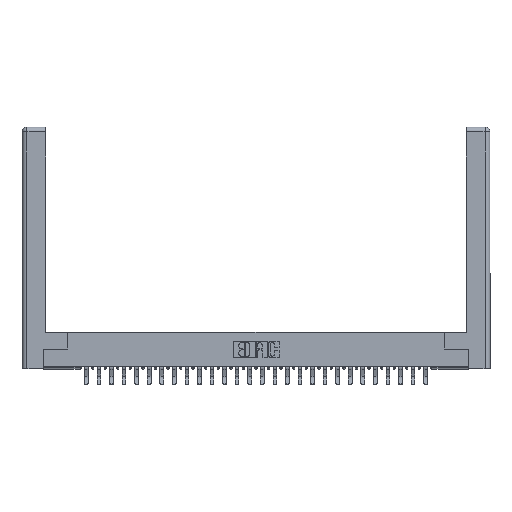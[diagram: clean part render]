
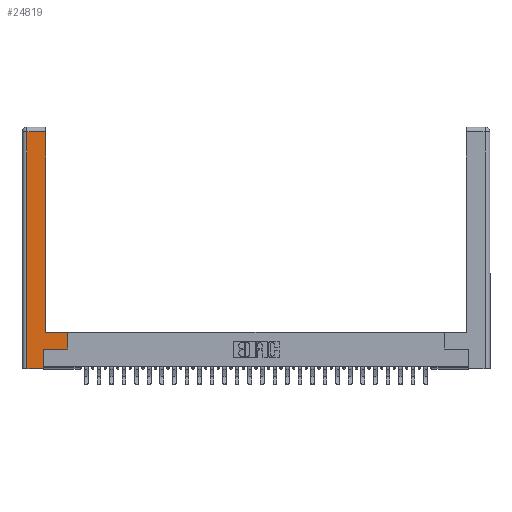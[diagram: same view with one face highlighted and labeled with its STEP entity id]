
A CAD part, top view. The second image highlights one B-rep face of the part: STEP entity #24819.
In plain terms, the highlighted planar face has unit normal (0, 0, 1).
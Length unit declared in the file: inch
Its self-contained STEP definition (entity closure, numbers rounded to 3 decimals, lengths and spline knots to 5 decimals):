
#255 = FACE_OUTER_BOUND ( 'NONE', #34238, .T. ) ;
#526 = DIRECTION ( 'NONE',  ( 0., 0., -1. ) ) ;
#2604 = CARTESIAN_POINT ( 'NONE',  ( 0., 0., 0. ) ) ;
#2842 = VECTOR ( 'NONE', #16489, 39.37008 ) ;
#3106 = ORIENTED_EDGE ( 'NONE', *, *, #4891, .T. ) ;
#4141 = CARTESIAN_POINT ( 'NONE',  ( 0.565, 0.45, 0. ) ) ;
#4891 = EDGE_CURVE ( 'NONE', #26411, #34265, #20602, .T. ) ;
#5141 = DIRECTION ( 'NONE',  ( -1., 0., 0. ) ) ;
#5194 = VERTEX_POINT ( 'NONE', #5573 ) ;
#5537 = PLANE ( 'NONE',  #10053 ) ;
#5573 = CARTESIAN_POINT ( 'NONE',  ( 0.565, 0.245, 0. ) ) ;
#6093 = VECTOR ( 'NONE', #22585, 39.37008 ) ;
#6288 = CARTESIAN_POINT ( 'NONE',  ( 0.295, 0.45, 0. ) ) ;
#7735 = CARTESIAN_POINT ( 'NONE',  ( 0.295, 0.45, 0. ) ) ;
#8131 = CARTESIAN_POINT ( 'NONE',  ( 0.0615, 0., 0. ) ) ;
#9075 = ORIENTED_EDGE ( 'NONE', *, *, #29049, .T. ) ;
#9185 = VECTOR ( 'NONE', #31605, 39.37008 ) ;
#9565 = CARTESIAN_POINT ( 'NONE',  ( 0.0615, 2.94, 0. ) ) ;
#10053 = AXIS2_PLACEMENT_3D ( 'NONE', #2604, #526, #26789 ) ;
#10129 = VERTEX_POINT ( 'NONE', #15245 ) ;
#10498 = LINE ( 'NONE', #4141, #15585 ) ;
#11147 = ORIENTED_EDGE ( 'NONE', *, *, #16006, .T. ) ;
#11263 = CARTESIAN_POINT ( 'NONE',  ( 0.295, 2.94, 0. ) ) ;
#12199 = ORIENTED_EDGE ( 'NONE', *, *, #34478, .T. ) ;
#12712 = CARTESIAN_POINT ( 'NONE',  ( 0.565, 0.245, 0. ) ) ;
#14322 = CARTESIAN_POINT ( 'NONE',  ( 0.0615, 0., 0. ) ) ;
#14647 = LINE ( 'NONE', #8131, #2842 ) ;
#14745 = CARTESIAN_POINT ( 'NONE',  ( 0.265, 0.245, 0. ) ) ;
#15245 = CARTESIAN_POINT ( 'NONE',  ( 0.565, 0.45, 0. ) ) ;
#15457 = EDGE_CURVE ( 'NONE', #34265, #28765, #17475, .T. ) ;
#15585 = VECTOR ( 'NONE', #33820, 39.37008 ) ;
#15619 = VERTEX_POINT ( 'NONE', #32944 ) ;
#16006 = EDGE_CURVE ( 'NONE', #10129, #26411, #21286, .T. ) ;
#16489 = DIRECTION ( 'NONE',  ( 0., -1., 0. ) ) ;
#17475 = LINE ( 'NONE', #27218, #27204 ) ;
#17507 = VECTOR ( 'NONE', #25610, 39.37008 ) ;
#20602 = LINE ( 'NONE', #23184, #9185 ) ;
#21286 = LINE ( 'NONE', #6288, #6093 ) ;
#21310 = LINE ( 'NONE', #31481, #30556 ) ;
#21412 = ORIENTED_EDGE ( 'NONE', *, *, #22362, .T. ) ;
#22362 = EDGE_CURVE ( 'NONE', #15619, #5194, #26170, .T. ) ;
#22585 = DIRECTION ( 'NONE',  ( -1., 0., 0. ) ) ;
#23184 = CARTESIAN_POINT ( 'NONE',  ( 0.295, 3., 0. ) ) ;
#24688 = LINE ( 'NONE', #14745, #17507 ) ;
#24819 = ADVANCED_FACE ( 'NONE', ( #255 ), #5537, .F. ) ;
#25146 = VERTEX_POINT ( 'NONE', #27817 ) ;
#25610 = DIRECTION ( 'NONE',  ( 0., 1., 0. ) ) ;
#26170 = LINE ( 'NONE', #12712, #34563 ) ;
#26411 = VERTEX_POINT ( 'NONE', #7735 ) ;
#26789 = DIRECTION ( 'NONE',  ( -1., 0., 0. ) ) ;
#27204 = VECTOR ( 'NONE', #5141, 39.37008 ) ;
#27218 = CARTESIAN_POINT ( 'NONE',  ( 0.0615, 2.94, 0. ) ) ;
#27817 = CARTESIAN_POINT ( 'NONE',  ( 0.265, 0., 0. ) ) ;
#27927 = ORIENTED_EDGE ( 'NONE', *, *, #15457, .T. ) ;
#28765 = VERTEX_POINT ( 'NONE', #9565 ) ;
#29049 = EDGE_CURVE ( 'NONE', #28765, #29934, #14647, .T. ) ;
#29934 = VERTEX_POINT ( 'NONE', #14322 ) ;
#30076 = ORIENTED_EDGE ( 'NONE', *, *, #31438, .T. ) ;
#30556 = VECTOR ( 'NONE', #31589, 39.37008 ) ;
#30596 = EDGE_CURVE ( 'NONE', #25146, #15619, #24688, .T. ) ;
#31438 = EDGE_CURVE ( 'NONE', #29934, #25146, #21310, .T. ) ;
#31481 = CARTESIAN_POINT ( 'NONE',  ( 0.265, 0., 0. ) ) ;
#31589 = DIRECTION ( 'NONE',  ( 1., 0., 0. ) ) ;
#31605 = DIRECTION ( 'NONE',  ( 0., 1., 0. ) ) ;
#32044 = ORIENTED_EDGE ( 'NONE', *, *, #30596, .T. ) ;
#32944 = CARTESIAN_POINT ( 'NONE',  ( 0.265, 0.245, 0. ) ) ;
#33664 = DIRECTION ( 'NONE',  ( 1., 0., 0. ) ) ;
#33820 = DIRECTION ( 'NONE',  ( 0., 1., 0. ) ) ;
#34238 = EDGE_LOOP ( 'NONE', ( #3106, #27927, #9075, #30076, #32044, #21412, #12199, #11147 ) ) ;
#34265 = VERTEX_POINT ( 'NONE', #11263 ) ;
#34478 = EDGE_CURVE ( 'NONE', #5194, #10129, #10498, .T. ) ;
#34563 = VECTOR ( 'NONE', #33664, 39.37008 ) ;
